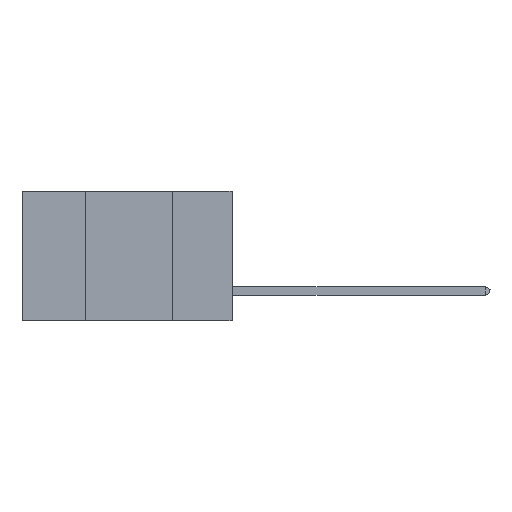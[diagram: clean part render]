
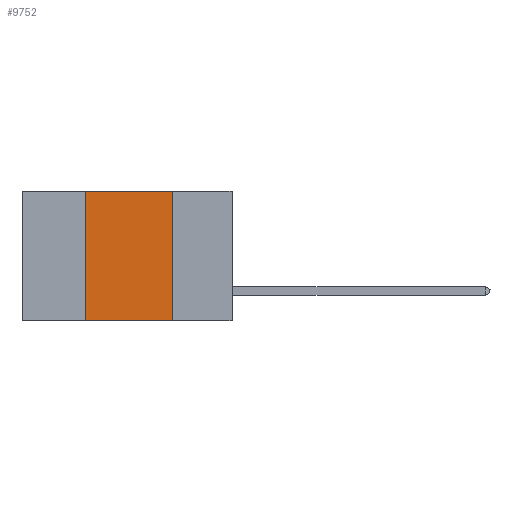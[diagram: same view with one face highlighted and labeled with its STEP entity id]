
A CAD part, left-side view. The second image highlights one B-rep face of the part: STEP entity #9752.
In plain terms, the highlighted planar face has unit normal (-1, 0, 0).
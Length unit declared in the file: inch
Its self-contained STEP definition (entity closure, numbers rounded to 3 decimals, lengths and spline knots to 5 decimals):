
#566 = CARTESIAN_POINT ( 'NONE',  ( 0., 0.17, -0.37 ) ) ;
#572 = EDGE_CURVE ( 'NONE', #8296, #15949, #15495, .T. ) ;
#895 = CARTESIAN_POINT ( 'NONE',  ( 0., 0.6, -0.37 ) ) ;
#963 = ORIENTED_EDGE ( 'NONE', *, *, #572, .F. ) ;
#1679 = ORIENTED_EDGE ( 'NONE', *, *, #2243, .F. ) ;
#2243 = EDGE_CURVE ( 'NONE', #14980, #3239, #11802, .T. ) ;
#2323 = FACE_OUTER_BOUND ( 'NONE', #7469, .T. ) ;
#3239 = VERTEX_POINT ( 'NONE', #566 ) ;
#4162 = LINE ( 'NONE', #4618, #16045 ) ;
#4596 = CARTESIAN_POINT ( 'NONE',  ( 0., 0.42, 0. ) ) ;
#4618 = CARTESIAN_POINT ( 'NONE',  ( 0., 0.6, 0. ) ) ;
#4634 = CARTESIAN_POINT ( 'NONE',  ( 0., 0.17, 0. ) ) ;
#6081 = VECTOR ( 'NONE', #16052, 39.37008 ) ;
#7368 = ORIENTED_EDGE ( 'NONE', *, *, #15073, .F. ) ;
#7469 = EDGE_LOOP ( 'NONE', ( #1679, #7368, #963, #16341 ) ) ;
#8296 = VERTEX_POINT ( 'NONE', #13969 ) ;
#9089 = VECTOR ( 'NONE', #10477, 39.37008 ) ;
#9122 = AXIS2_PLACEMENT_3D ( 'NONE', #13861, #16315, #15862 ) ;
#9752 = ADVANCED_FACE ( 'NONE', ( #2323 ), #10136, .F. ) ;
#10136 = PLANE ( 'NONE',  #9122 ) ;
#10477 = DIRECTION ( 'NONE',  ( 0., -1., 0. ) ) ;
#11802 = LINE ( 'NONE', #13219, #6081 ) ;
#11867 = VECTOR ( 'NONE', #14081, 39.37008 ) ;
#12692 = DIRECTION ( 'NONE',  ( 0., -1., 0. ) ) ;
#12739 = LINE ( 'NONE', #895, #9089 ) ;
#13000 = CARTESIAN_POINT ( 'NONE',  ( 0., 0.42, 0. ) ) ;
#13219 = CARTESIAN_POINT ( 'NONE',  ( 0., 0.17, 0. ) ) ;
#13336 = EDGE_CURVE ( 'NONE', #8296, #3239, #12739, .T. ) ;
#13861 = CARTESIAN_POINT ( 'NONE',  ( 0., 0.6, 0. ) ) ;
#13969 = CARTESIAN_POINT ( 'NONE',  ( 0., 0.42, -0.37 ) ) ;
#14081 = DIRECTION ( 'NONE',  ( 0., 0., 1. ) ) ;
#14980 = VERTEX_POINT ( 'NONE', #4634 ) ;
#15073 = EDGE_CURVE ( 'NONE', #15949, #14980, #4162, .T. ) ;
#15495 = LINE ( 'NONE', #4596, #11867 ) ;
#15862 = DIRECTION ( 'NONE',  ( 0., 0., -1. ) ) ;
#15949 = VERTEX_POINT ( 'NONE', #13000 ) ;
#16045 = VECTOR ( 'NONE', #12692, 39.37008 ) ;
#16052 = DIRECTION ( 'NONE',  ( 0., 0., -1. ) ) ;
#16315 = DIRECTION ( 'NONE',  ( 1., 0., 0. ) ) ;
#16341 = ORIENTED_EDGE ( 'NONE', *, *, #13336, .T. ) ;
